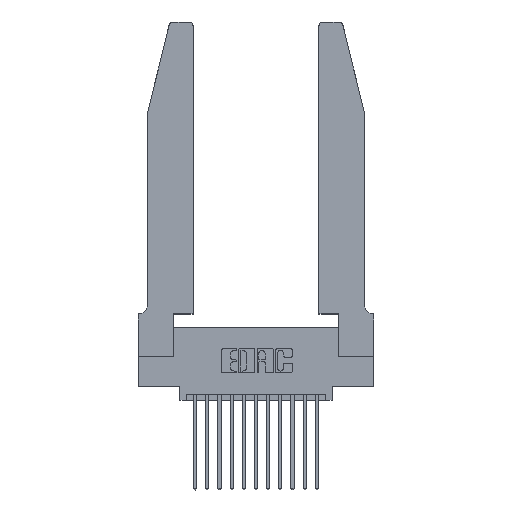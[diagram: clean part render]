
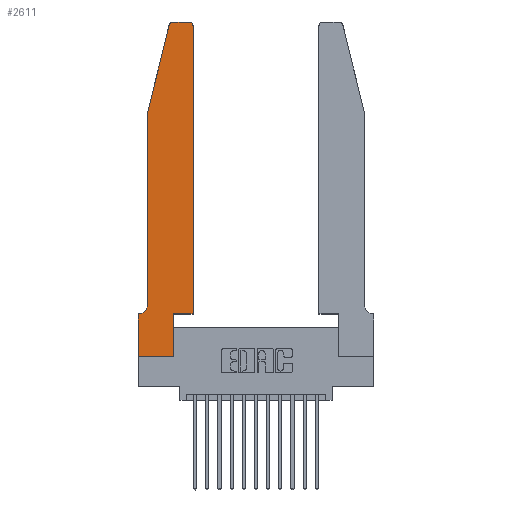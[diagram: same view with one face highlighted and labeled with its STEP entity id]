
A CAD part, top view. The second image highlights one B-rep face of the part: STEP entity #2611.
In plain terms, the highlighted planar face has unit normal (0, 0, 1).
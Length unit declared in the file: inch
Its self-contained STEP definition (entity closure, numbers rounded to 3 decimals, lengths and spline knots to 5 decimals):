
#221 = CARTESIAN_POINT ( 'NONE',  ( 0.0055, 0.42, 0.37 ) ) ;
#419 = VERTEX_POINT ( 'NONE', #9280 ) ;
#481 = CARTESIAN_POINT ( 'NONE',  ( 0., 0., 0.37 ) ) ;
#564 = EDGE_CURVE ( 'NONE', #2111, #6764, #15545, .T. ) ;
#687 = CARTESIAN_POINT ( 'NONE',  ( 0.25487, 2.72718, 0.37 ) ) ;
#942 = LINE ( 'NONE', #17497, #16555 ) ;
#956 = DIRECTION ( 'NONE',  ( 0., 0., 1. ) ) ;
#1002 = VERTEX_POINT ( 'NONE', #16011 ) ;
#1386 = ORIENTED_EDGE ( 'NONE', *, *, #2341, .T. ) ;
#1462 = VECTOR ( 'NONE', #2526, 39.37008 ) ;
#1584 = LINE ( 'NONE', #3386, #10546 ) ;
#1616 = LINE ( 'NONE', #6653, #3315 ) ;
#1722 = DIRECTION ( 'NONE',  ( -1., 0., 0. ) ) ;
#1853 = EDGE_CURVE ( 'NONE', #8097, #1002, #1616, .T. ) ;
#1985 = CARTESIAN_POINT ( 'NONE',  ( 0.2865, 0.35, 0.37 ) ) ;
#2111 = VERTEX_POINT ( 'NONE', #11770 ) ;
#2341 = EDGE_CURVE ( 'NONE', #2502, #2111, #9724, .T. ) ;
#2448 = CARTESIAN_POINT ( 'NONE',  ( 0.0055, 0.35, 0.37 ) ) ;
#2502 = VERTEX_POINT ( 'NONE', #1985 ) ;
#2526 = DIRECTION ( 'NONE',  ( -0.239, -0.971, 0. ) ) ;
#2572 = CARTESIAN_POINT ( 'NONE',  ( 0.4505, 0.35, 0.37 ) ) ;
#2611 = ADVANCED_FACE ( 'NONE', ( #10540 ), #13095, .T. ) ;
#2682 = DIRECTION ( 'NONE',  ( 0., 0., 1. ) ) ;
#2962 = EDGE_CURVE ( 'NONE', #5037, #12621, #13072, .T. ) ;
#3315 = VECTOR ( 'NONE', #16285, 39.37008 ) ;
#3386 = CARTESIAN_POINT ( 'NONE',  ( 0., 0., 0.37 ) ) ;
#3420 = EDGE_CURVE ( 'NONE', #1002, #6409, #13468, .T. ) ;
#3549 = AXIS2_PLACEMENT_3D ( 'NONE', #10922, #2682, #8146 ) ;
#4061 = DIRECTION ( 'NONE',  ( 1., 0., 0. ) ) ;
#4507 = CARTESIAN_POINT ( 'NONE',  ( 0., 0.35, 0.37 ) ) ;
#4562 = EDGE_CURVE ( 'NONE', #6764, #8097, #11516, .T. ) ;
#4904 = CARTESIAN_POINT ( 'NONE',  ( 0., 0.35, 0.37 ) ) ;
#5037 = VERTEX_POINT ( 'NONE', #16877 ) ;
#5142 = CARTESIAN_POINT ( 'NONE',  ( 0.2865, 0., 0.37 ) ) ;
#5225 = ORIENTED_EDGE ( 'NONE', *, *, #11864, .T. ) ;
#5300 = CARTESIAN_POINT ( 'NONE',  ( 0.284, 2.72, 0.37 ) ) ;
#5389 = ORIENTED_EDGE ( 'NONE', *, *, #9864, .T. ) ;
#6409 = VERTEX_POINT ( 'NONE', #687 ) ;
#6511 = LINE ( 'NONE', #17098, #11209 ) ;
#6653 = CARTESIAN_POINT ( 'NONE',  ( 0.2605, 2.75, 0.37 ) ) ;
#6764 = VERTEX_POINT ( 'NONE', #15314 ) ;
#6857 = AXIS2_PLACEMENT_3D ( 'NONE', #4904, #956, #7721 ) ;
#7035 = CARTESIAN_POINT ( 'NONE',  ( 0.4205, 2.75, 0.37 ) ) ;
#7143 = VERTEX_POINT ( 'NONE', #5142 ) ;
#7179 = DIRECTION ( 'NONE',  ( 0., 0., -1. ) ) ;
#7254 = LINE ( 'NONE', #9291, #1462 ) ;
#7639 = EDGE_CURVE ( 'NONE', #419, #7143, #17419, .T. ) ;
#7721 = DIRECTION ( 'NONE',  ( 1., 0., 0. ) ) ;
#7766 = EDGE_CURVE ( 'NONE', #13425, #419, #1584, .T. ) ;
#8097 = VERTEX_POINT ( 'NONE', #7035 ) ;
#8146 = DIRECTION ( 'NONE',  ( 1., 0., 0. ) ) ;
#8159 = VECTOR ( 'NONE', #15222, 39.37008 ) ;
#8173 = ORIENTED_EDGE ( 'NONE', *, *, #14133, .T. ) ;
#8287 = CARTESIAN_POINT ( 'NONE',  ( 0.4505, 0.35, 0.37 ) ) ;
#8399 = DIRECTION ( 'NONE',  ( 0., 1., 0. ) ) ;
#8914 = DIRECTION ( 'NONE',  ( -1., 0., 0. ) ) ;
#9032 = AXIS2_PLACEMENT_3D ( 'NONE', #221, #7179, #1722 ) ;
#9280 = CARTESIAN_POINT ( 'NONE',  ( 0., 0., 0.37 ) ) ;
#9291 = CARTESIAN_POINT ( 'NONE',  ( 0.0755, 2., 0.37 ) ) ;
#9724 = LINE ( 'NONE', #2572, #15499 ) ;
#9864 = EDGE_CURVE ( 'NONE', #7143, #2502, #12642, .T. ) ;
#10255 = DIRECTION ( 'NONE',  ( 0., -1., 0. ) ) ;
#10319 = EDGE_LOOP ( 'NONE', ( #16543, #10499, #5225, #10865, #11729, #8173, #15664, #12911, #5389, #1386, #15911, #15840 ) ) ;
#10499 = ORIENTED_EDGE ( 'NONE', *, *, #3420, .T. ) ;
#10540 = FACE_OUTER_BOUND ( 'NONE', #10319, .T. ) ;
#10546 = VECTOR ( 'NONE', #10255, 39.37008 ) ;
#10841 = DIRECTION ( 'NONE',  ( 0., 0., 1. ) ) ;
#10865 = ORIENTED_EDGE ( 'NONE', *, *, #14417, .T. ) ;
#10898 = DIRECTION ( 'NONE',  ( 1., 0., 0. ) ) ;
#10922 = CARTESIAN_POINT ( 'NONE',  ( 0.4205, 2.72, 0.37 ) ) ;
#11209 = VECTOR ( 'NONE', #8914, 39.37008 ) ;
#11337 = CARTESIAN_POINT ( 'NONE',  ( 0.0755, 2., 0.37 ) ) ;
#11516 = CIRCLE ( 'NONE', #3549, 0.03 ) ;
#11729 = ORIENTED_EDGE ( 'NONE', *, *, #2962, .T. ) ;
#11770 = CARTESIAN_POINT ( 'NONE',  ( 0.4505, 0.35, 0.37 ) ) ;
#11864 = EDGE_CURVE ( 'NONE', #6409, #12928, #7254, .T. ) ;
#12613 = DIRECTION ( 'NONE',  ( 1., 0., 0. ) ) ;
#12621 = VERTEX_POINT ( 'NONE', #2448 ) ;
#12642 = LINE ( 'NONE', #15346, #8159 ) ;
#12911 = ORIENTED_EDGE ( 'NONE', *, *, #7639, .T. ) ;
#12928 = VERTEX_POINT ( 'NONE', #11337 ) ;
#13072 = CIRCLE ( 'NONE', #9032, 0.07 ) ;
#13095 = PLANE ( 'NONE',  #6857 ) ;
#13425 = VERTEX_POINT ( 'NONE', #4507 ) ;
#13468 = CIRCLE ( 'NONE', #15688, 0.03 ) ;
#13777 = VECTOR ( 'NONE', #12613, 39.37008 ) ;
#14133 = EDGE_CURVE ( 'NONE', #12621, #13425, #6511, .T. ) ;
#14417 = EDGE_CURVE ( 'NONE', #12928, #5037, #942, .T. ) ;
#14793 = DIRECTION ( 'NONE',  ( 0., -1., 0. ) ) ;
#15222 = DIRECTION ( 'NONE',  ( 0., 1., 0. ) ) ;
#15314 = CARTESIAN_POINT ( 'NONE',  ( 0.4505, 2.72, 0.37 ) ) ;
#15346 = CARTESIAN_POINT ( 'NONE',  ( 0.2865, 0.35, 0.37 ) ) ;
#15499 = VECTOR ( 'NONE', #4061, 39.37008 ) ;
#15545 = LINE ( 'NONE', #8287, #15758 ) ;
#15664 = ORIENTED_EDGE ( 'NONE', *, *, #7766, .T. ) ;
#15688 = AXIS2_PLACEMENT_3D ( 'NONE', #5300, #10841, #10898 ) ;
#15758 = VECTOR ( 'NONE', #8399, 39.37008 ) ;
#15840 = ORIENTED_EDGE ( 'NONE', *, *, #4562, .T. ) ;
#15911 = ORIENTED_EDGE ( 'NONE', *, *, #564, .T. ) ;
#16011 = CARTESIAN_POINT ( 'NONE',  ( 0.284, 2.75, 0.37 ) ) ;
#16285 = DIRECTION ( 'NONE',  ( -1., 0., 0. ) ) ;
#16543 = ORIENTED_EDGE ( 'NONE', *, *, #1853, .T. ) ;
#16555 = VECTOR ( 'NONE', #14793, 39.37008 ) ;
#16877 = CARTESIAN_POINT ( 'NONE',  ( 0.0755, 0.42, 0.37 ) ) ;
#17098 = CARTESIAN_POINT ( 'NONE',  ( 0.0755, 0.35, 0.37 ) ) ;
#17419 = LINE ( 'NONE', #481, #13777 ) ;
#17497 = CARTESIAN_POINT ( 'NONE',  ( 0.0755, 2., 0.37 ) ) ;
